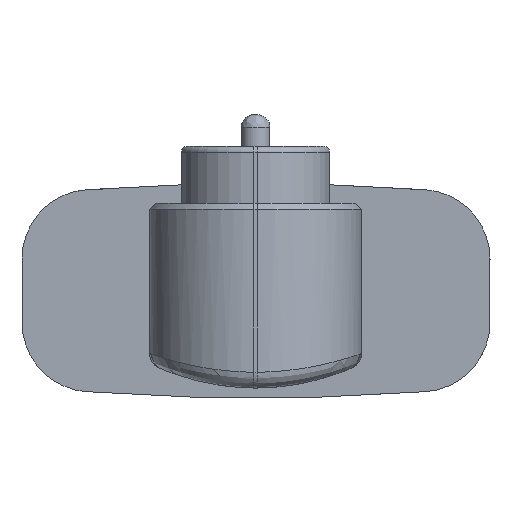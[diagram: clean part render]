
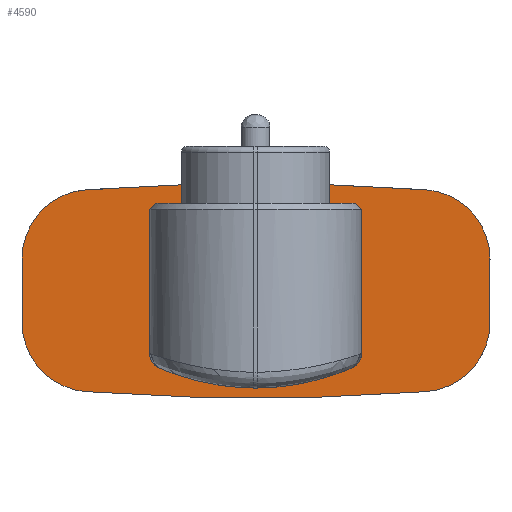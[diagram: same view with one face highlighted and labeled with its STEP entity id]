
A CAD part, left-side view. The second image highlights one B-rep face of the part: STEP entity #4590.
In plain terms, the highlighted planar face has unit normal (-1, 0, 0).
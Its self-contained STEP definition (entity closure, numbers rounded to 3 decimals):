
#45 = CIRCLE ( 'NONE', #8068, 2.75 ) ;
#438 = ORIENTED_EDGE ( 'NONE', *, *, #1770, .T. ) ;
#696 = VERTEX_POINT ( 'NONE', #8716 ) ;
#747 = AXIS2_PLACEMENT_3D ( 'NONE', #2081, #5478, #8320 ) ;
#941 = ORIENTED_EDGE ( 'NONE', *, *, #4518, .F. ) ;
#942 = DIRECTION ( 'NONE',  ( -1., 0., 0. ) ) ;
#1113 = ORIENTED_EDGE ( 'NONE', *, *, #8092, .F. ) ;
#1375 = VERTEX_POINT ( 'NONE', #8277 ) ;
#1620 = AXIS2_PLACEMENT_3D ( 'NONE', #8503, #6871, #10689 ) ;
#1655 = VERTEX_POINT ( 'NONE', #6049 ) ;
#1753 = EDGE_CURVE ( 'NONE', #696, #1655, #1926, .T. ) ;
#1770 = EDGE_CURVE ( 'NONE', #3279, #9258, #45, .T. ) ;
#1805 = CIRCLE ( 'NONE', #10236, 2.75 ) ;
#1824 = DIRECTION ( 'NONE',  ( 0., 1., 0. ) ) ;
#1926 = CIRCLE ( 'NONE', #5092, 2.2 ) ;
#1929 = ORIENTED_EDGE ( 'NONE', *, *, #5444, .T. ) ;
#2081 = CARTESIAN_POINT ( 'NONE',  ( 83.6, -0.015, 62.029 ) ) ;
#2103 = CARTESIAN_POINT ( 'NONE',  ( 83.6, -5.379, -7.765 ) ) ;
#2276 = DIRECTION ( 'NONE',  ( -1., 0., 0. ) ) ;
#2358 = EDGE_CURVE ( 'NONE', #7703, #9918, #9667, .T. ) ;
#2394 = VERTEX_POINT ( 'NONE', #2103 ) ;
#2594 = DIRECTION ( 'NONE',  ( -1., 0., 0. ) ) ;
#2767 = DIRECTION ( 'NONE',  ( 0., 1., 0. ) ) ;
#2793 = CIRCLE ( 'NONE', #747, 70. ) ;
#2813 = CARTESIAN_POINT ( 'NONE',  ( 83.6, 5.185, -3.571 ) ) ;
#3136 = FACE_BOUND ( 'NONE', #5533, .T. ) ;
#3279 = VERTEX_POINT ( 'NONE', #3768 ) ;
#3301 = PLANE ( 'NONE',  #1620 ) ;
#3376 = CARTESIAN_POINT ( 'NONE',  ( 83.6, 5.352, -1.377 ) ) ;
#3382 = CARTESIAN_POINT ( 'NONE',  ( 83.6, -0.015, -4.571 ) ) ;
#3524 = FACE_OUTER_BOUND ( 'NONE', #7590, .T. ) ;
#3679 = CARTESIAN_POINT ( 'NONE',  ( 83.6, 7.385, -5.571 ) ) ;
#3742 = DIRECTION ( 'NONE',  ( 0., 1., 0. ) ) ;
#3768 = CARTESIAN_POINT ( 'NONE',  ( 83.6, -2.765, -4.571 ) ) ;
#4178 = DIRECTION ( 'NONE',  ( 1., 0., 0. ) ) ;
#4251 = DIRECTION ( 'NONE',  ( 1., 0., 0. ) ) ;
#4291 = AXIS2_PLACEMENT_3D ( 'NONE', #6155, #4178, #9750 ) ;
#4490 = EDGE_CURVE ( 'NONE', #1655, #7703, #10846, .T. ) ;
#4518 = EDGE_CURVE ( 'NONE', #1375, #5751, #7284, .T. ) ;
#4590 = ADVANCED_FACE ( 'NONE', ( #3524, #3136 ), #3301, .T. ) ;
#4603 = AXIS2_PLACEMENT_3D ( 'NONE', #2813, #7422, #3742 ) ;
#4849 = EDGE_CURVE ( 'NONE', #9918, #5751, #7732, .T. ) ;
#5092 = AXIS2_PLACEMENT_3D ( 'NONE', #11168, #2276, #2767 ) ;
#5179 = DIRECTION ( 'NONE',  ( 0., 0., -1. ) ) ;
#5229 = DIRECTION ( 'NONE',  ( 0., 0., 1. ) ) ;
#5293 = CARTESIAN_POINT ( 'NONE',  ( 83.6, 7.385, -3.571 ) ) ;
#5344 = VECTOR ( 'NONE', #5179, 1000. ) ;
#5444 = EDGE_CURVE ( 'NONE', #9258, #3279, #1805, .T. ) ;
#5478 = DIRECTION ( 'NONE',  ( 1., 0., 0. ) ) ;
#5533 = EDGE_LOOP ( 'NONE', ( #438, #1929 ) ) ;
#5751 = VERTEX_POINT ( 'NONE', #3679 ) ;
#6049 = CARTESIAN_POINT ( 'NONE',  ( 83.6, -5.383, -1.377 ) ) ;
#6155 = CARTESIAN_POINT ( 'NONE',  ( 83.6, 5.185, -5.571 ) ) ;
#6855 = LINE ( 'NONE', #10631, #7280 ) ;
#6871 = DIRECTION ( 'NONE',  ( -1., 0., 0. ) ) ;
#7060 = CARTESIAN_POINT ( 'NONE',  ( 83.6, 2.735, -4.571 ) ) ;
#7280 = VECTOR ( 'NONE', #5229, 1000. ) ;
#7284 = CIRCLE ( 'NONE', #4291, 2.2 ) ;
#7290 = ORIENTED_EDGE ( 'NONE', *, *, #4490, .T. ) ;
#7422 = DIRECTION ( 'NONE',  ( -1., 0., 0. ) ) ;
#7590 = EDGE_LOOP ( 'NONE', ( #11445, #9040, #941, #1113, #8097, #8296, #9276, #7290 ) ) ;
#7626 = CARTESIAN_POINT ( 'NONE',  ( 83.6, -0.015, -71.171 ) ) ;
#7703 = VERTEX_POINT ( 'NONE', #3376 ) ;
#7723 = CARTESIAN_POINT ( 'NONE',  ( 83.6, -7.415, -5.571 ) ) ;
#7732 = LINE ( 'NONE', #8804, #5344 ) ;
#7828 = AXIS2_PLACEMENT_3D ( 'NONE', #7626, #2594, #9400 ) ;
#8052 = DIRECTION ( 'NONE',  ( 0., 1., 0. ) ) ;
#8068 = AXIS2_PLACEMENT_3D ( 'NONE', #3382, #4251, #11227 ) ;
#8092 = EDGE_CURVE ( 'NONE', #2394, #1375, #2793, .T. ) ;
#8097 = ORIENTED_EDGE ( 'NONE', *, *, #8929, .T. ) ;
#8170 = CIRCLE ( 'NONE', #9696, 2.2 ) ;
#8277 = CARTESIAN_POINT ( 'NONE',  ( 83.6, 5.354, -7.765 ) ) ;
#8296 = ORIENTED_EDGE ( 'NONE', *, *, #11017, .T. ) ;
#8320 = DIRECTION ( 'NONE',  ( 0., 1., 0. ) ) ;
#8503 = CARTESIAN_POINT ( 'NONE',  ( 83.6, -0.015, -4.571 ) ) ;
#8716 = CARTESIAN_POINT ( 'NONE',  ( 83.6, -7.415, -3.571 ) ) ;
#8804 = CARTESIAN_POINT ( 'NONE',  ( 83.6, 7.385, -4.571 ) ) ;
#8929 = EDGE_CURVE ( 'NONE', #2394, #10132, #8170, .T. ) ;
#8946 = CARTESIAN_POINT ( 'NONE',  ( 83.6, -5.215, -5.571 ) ) ;
#8960 = CARTESIAN_POINT ( 'NONE',  ( 83.6, -0.015, -4.571 ) ) ;
#9040 = ORIENTED_EDGE ( 'NONE', *, *, #4849, .T. ) ;
#9258 = VERTEX_POINT ( 'NONE', #7060 ) ;
#9276 = ORIENTED_EDGE ( 'NONE', *, *, #1753, .T. ) ;
#9400 = DIRECTION ( 'NONE',  ( 0., 1., 0. ) ) ;
#9667 = CIRCLE ( 'NONE', #4603, 2.2 ) ;
#9696 = AXIS2_PLACEMENT_3D ( 'NONE', #8946, #942, #8052 ) ;
#9750 = DIRECTION ( 'NONE',  ( 0., 1., 0. ) ) ;
#9918 = VERTEX_POINT ( 'NONE', #5293 ) ;
#9961 = DIRECTION ( 'NONE',  ( 1., 0., 0. ) ) ;
#10132 = VERTEX_POINT ( 'NONE', #7723 ) ;
#10236 = AXIS2_PLACEMENT_3D ( 'NONE', #8960, #9961, #1824 ) ;
#10631 = CARTESIAN_POINT ( 'NONE',  ( 83.6, -7.415, -4.571 ) ) ;
#10689 = DIRECTION ( 'NONE',  ( 0., 1., 0. ) ) ;
#10846 = CIRCLE ( 'NONE', #7828, 70. ) ;
#11017 = EDGE_CURVE ( 'NONE', #10132, #696, #6855, .T. ) ;
#11168 = CARTESIAN_POINT ( 'NONE',  ( 83.6, -5.215, -3.571 ) ) ;
#11227 = DIRECTION ( 'NONE',  ( 0., 1., 0. ) ) ;
#11445 = ORIENTED_EDGE ( 'NONE', *, *, #2358, .T. ) ;
